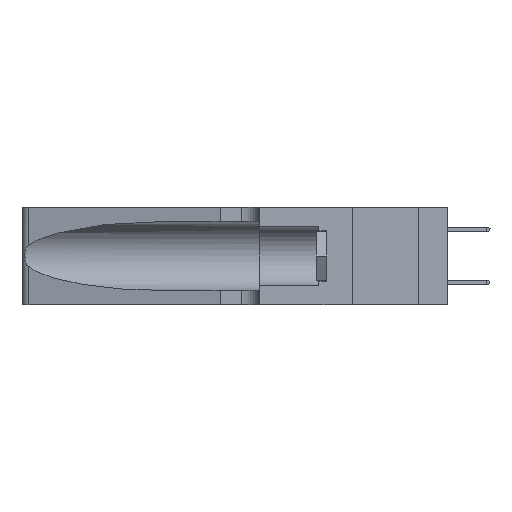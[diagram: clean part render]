
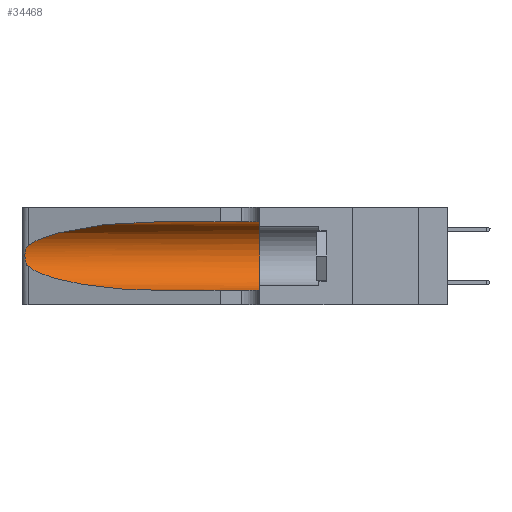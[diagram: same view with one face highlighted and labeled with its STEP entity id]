
A CAD part, left-side view. The second image highlights one B-rep face of the part: STEP entity #34468.
In plain terms, the highlighted cylindrical face has radius 3.308 mm (diameter 6.617 mm), a partial arc.
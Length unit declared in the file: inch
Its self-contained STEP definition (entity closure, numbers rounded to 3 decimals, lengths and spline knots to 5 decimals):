
#51 = AXIS2_PLACEMENT_3D ( 'NONE', #2489, #5410, #11052 ) ;
#966 = CARTESIAN_POINT ( 'NONE',  ( 0.25487, 1.22718, 0.14631 ) ) ;
#1064 = CARTESIAN_POINT ( 'NONE',  ( 0.25555, 1.22994, 0.2215 ) ) ;
#1173 = AXIS2_PLACEMENT_3D ( 'NONE', #36467, #33428, #24700 ) ;
#1300 = CARTESIAN_POINT ( 'NONE',  ( 0.25487, 1.22718, 0.22369 ) ) ;
#1698 = CARTESIAN_POINT ( 'NONE',  ( 0.1305, 0.72297, 0.31525 ) ) ;
#1797 = VECTOR ( 'NONE', #17463, 39.37008 ) ;
#2195 = FACE_OUTER_BOUND ( 'NONE', #20005, .T. ) ;
#2489 = CARTESIAN_POINT ( 'NONE',  ( 0.1305, 0.35, 0.185 ) ) ;
#2690 = CYLINDRICAL_SURFACE ( 'NONE', #1173, 0.13025 ) ;
#2922 = VERTEX_POINT ( 'NONE', #11499 ) ;
#3730 = VERTEX_POINT ( 'NONE', #32355 ) ;
#4029 = CARTESIAN_POINT ( 'NONE',  ( 0.26075, 1.23896, 0.19203 ) ) ;
#4977 = CARTESIAN_POINT ( 'NONE',  ( 0.18966, 0.96281, 0.05475 ) ) ;
#4978 =( BOUNDED_CURVE ( )  B_SPLINE_CURVE ( 3, ( #34242, #22553, #4977, #8162 ),
 .UNSPECIFIED., .F., .F. ) 
 B_SPLINE_CURVE_WITH_KNOTS ( ( 4, 4 ),
 ( 3.44316, 4.71239 ),
 .UNSPECIFIED. ) 
 CURVE ( )  GEOMETRIC_REPRESENTATION_ITEM ( )  RATIONAL_B_SPLINE_CURVE ( ( 1., 0.87, 0.87, 1. ) ) 
 REPRESENTATION_ITEM ( '' )  );
#5410 = DIRECTION ( 'NONE',  ( 0., 1., 0. ) ) ;
#5672 = ORIENTED_EDGE ( 'NONE', *, *, #26309, .T. ) ;
#6277 = EDGE_CURVE ( 'NONE', #13941, #14869, #7291, .T. ) ;
#6387 = ORIENTED_EDGE ( 'NONE', *, *, #36966, .T. ) ;
#6451 = ORIENTED_EDGE ( 'NONE', *, *, #25900, .T. ) ;
#6796 = CARTESIAN_POINT ( 'NONE',  ( 0.1305, 0.72297, 0.31525 ) ) ;
#7291 = B_SPLINE_CURVE_WITH_KNOTS ( 'NONE', 3,
 ( #18892, #1064, #27647, #25225, #30992, #16466, #4029, #26183, #30871, #19127, #21611, #24269, #12947, #27252 ),
 .UNSPECIFIED., .F., .F.,
 ( 4, 2, 2, 2, 2, 2, 4 ),
 ( 0., 0.00027, 0.00053, 0.00107, 0.0016, 0.00187, 0.00214 ),
 .UNSPECIFIED. ) ;
#7886 = LINE ( 'NONE', #27620, #30865 ) ;
#8162 = CARTESIAN_POINT ( 'NONE',  ( 0.1305, 0.72297, 0.05475 ) ) ;
#11052 = DIRECTION ( 'NONE',  ( 0., 0., 1. ) ) ;
#11499 = CARTESIAN_POINT ( 'NONE',  ( 0.1305, 0.72297, 0.05475 ) ) ;
#12804 = EDGE_CURVE ( 'NONE', #19500, #3730, #7886, .T. ) ;
#12947 = CARTESIAN_POINT ( 'NONE',  ( 0.25555, 1.22993, 0.14849 ) ) ;
#13010 = VERTEX_POINT ( 'NONE', #15749 ) ;
#13941 = VERTEX_POINT ( 'NONE', #23537 ) ;
#14499 = CARTESIAN_POINT ( 'NONE',  ( 0.1305, 1.61858, 0.05475 ) ) ;
#14869 = VERTEX_POINT ( 'NONE', #966 ) ;
#15749 = CARTESIAN_POINT ( 'NONE',  ( 0.1305, 0.35, 0.05475 ) ) ;
#15799 = DIRECTION ( 'NONE',  ( 0., -1., 0. ) ) ;
#16466 = CARTESIAN_POINT ( 'NONE',  ( 0.26018, 1.23835, 0.19895 ) ) ;
#17463 = DIRECTION ( 'NONE',  ( 0., -1., 0. ) ) ;
#18892 = CARTESIAN_POINT ( 'NONE',  ( 0.25487, 1.22718, 0.22369 ) ) ;
#19127 = CARTESIAN_POINT ( 'NONE',  ( 0.25856, 1.23593, 0.16098 ) ) ;
#19500 = VERTEX_POINT ( 'NONE', #1698 ) ;
#19650 = EDGE_CURVE ( 'NONE', #3730, #13010, #32905, .T. ) ;
#20005 = EDGE_LOOP ( 'NONE', ( #6387, #27182, #5672, #6451, #36273, #31263 ) ) ;
#21611 = CARTESIAN_POINT ( 'NONE',  ( 0.25789, 1.23486, 0.15765 ) ) ;
#22553 = CARTESIAN_POINT ( 'NONE',  ( 0.2373, 1.15595, 0.08982 ) ) ;
#23537 = CARTESIAN_POINT ( 'NONE',  ( 0.25487, 1.22718, 0.22369 ) ) ;
#24269 = CARTESIAN_POINT ( 'NONE',  ( 0.25639, 1.23186, 0.15144 ) ) ;
#24700 = DIRECTION ( 'NONE',  ( 0., 0., -1. ) ) ;
#25225 = CARTESIAN_POINT ( 'NONE',  ( 0.25787, 1.23484, 0.2124 ) ) ;
#25900 = EDGE_CURVE ( 'NONE', #2922, #13010, #37600, .T. ) ;
#26183 = CARTESIAN_POINT ( 'NONE',  ( 0.26075, 1.23896, 0.178 ) ) ;
#26309 = EDGE_CURVE ( 'NONE', #14869, #2922, #4978, .T. ) ;
#27182 = ORIENTED_EDGE ( 'NONE', *, *, #6277, .T. ) ;
#27252 = CARTESIAN_POINT ( 'NONE',  ( 0.25487, 1.22718, 0.14631 ) ) ;
#27620 = CARTESIAN_POINT ( 'NONE',  ( 0.1305, 1.61858, 0.31525 ) ) ;
#27647 = CARTESIAN_POINT ( 'NONE',  ( 0.25639, 1.23184, 0.21858 ) ) ;
#30587 = CARTESIAN_POINT ( 'NONE',  ( 0.2373, 1.15595, 0.28018 ) ) ;
#30848 = CARTESIAN_POINT ( 'NONE',  ( 0.18966, 0.96281, 0.31525 ) ) ;
#30865 = VECTOR ( 'NONE', #15799, 39.37008 ) ;
#30871 = CARTESIAN_POINT ( 'NONE',  ( 0.26017, 1.23833, 0.17102 ) ) ;
#30992 = CARTESIAN_POINT ( 'NONE',  ( 0.25854, 1.2359, 0.20912 ) ) ;
#31263 = ORIENTED_EDGE ( 'NONE', *, *, #12804, .F. ) ;
#32355 = CARTESIAN_POINT ( 'NONE',  ( 0.1305, 0.35, 0.31525 ) ) ;
#32905 = CIRCLE ( 'NONE', #51, 0.13025 ) ;
#33428 = DIRECTION ( 'NONE',  ( 0., -1., 0. ) ) ;
#34148 =( BOUNDED_CURVE ( )  B_SPLINE_CURVE ( 3, ( #6796, #30848, #30587, #1300 ),
 .UNSPECIFIED., .F., .T. ) 
 B_SPLINE_CURVE_WITH_KNOTS ( ( 4, 4 ),
 ( 1.5708, 2.84003 ),
 .UNSPECIFIED. ) 
 CURVE ( )  GEOMETRIC_REPRESENTATION_ITEM ( )  RATIONAL_B_SPLINE_CURVE ( ( 1., 0.87, 0.87, 1. ) ) 
 REPRESENTATION_ITEM ( '' )  );
#34242 = CARTESIAN_POINT ( 'NONE',  ( 0.25487, 1.22718, 0.14631 ) ) ;
#34468 = ADVANCED_FACE ( 'NONE', ( #2195 ), #2690, .F. ) ;
#36273 = ORIENTED_EDGE ( 'NONE', *, *, #19650, .F. ) ;
#36467 = CARTESIAN_POINT ( 'NONE',  ( 0.1305, 1.61858, 0.185 ) ) ;
#36966 = EDGE_CURVE ( 'NONE', #19500, #13941, #34148, .T. ) ;
#37600 = LINE ( 'NONE', #14499, #1797 ) ;
